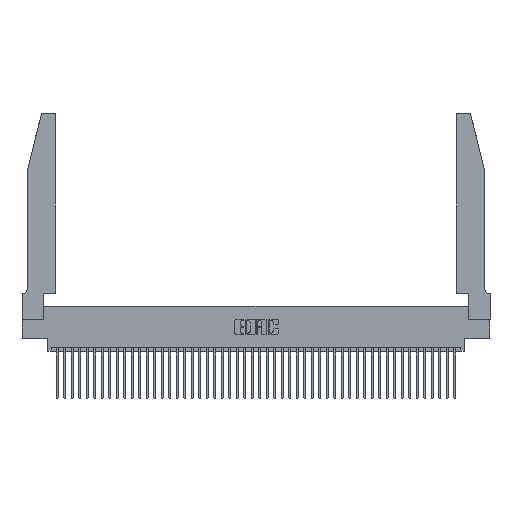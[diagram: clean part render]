
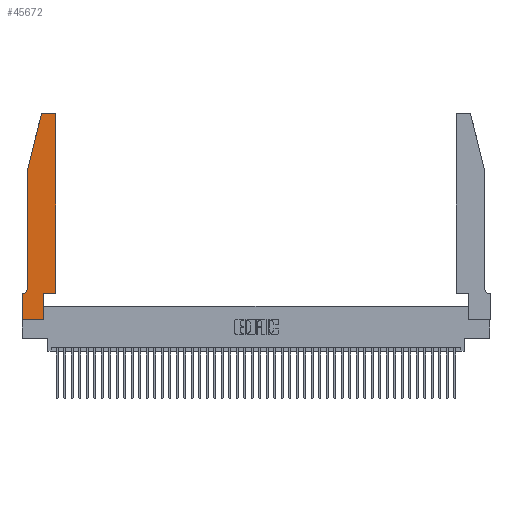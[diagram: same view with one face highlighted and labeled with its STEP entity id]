
A CAD part, top view. The second image highlights one B-rep face of the part: STEP entity #45672.
In plain terms, the highlighted planar face has unit normal (0, 0, 1).
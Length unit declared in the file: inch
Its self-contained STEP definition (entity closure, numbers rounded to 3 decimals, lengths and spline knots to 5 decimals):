
#486 = CARTESIAN_POINT ( 'NONE',  ( 0., 0., 0.37 ) ) ;
#1083 = EDGE_CURVE ( 'NONE', #6959, #23829, #30853, .T. ) ;
#2503 = EDGE_CURVE ( 'NONE', #8473, #39473, #43891, .T. ) ;
#3079 = VECTOR ( 'NONE', #40499, 39.37008 ) ;
#3240 = VECTOR ( 'NONE', #13297, 39.37008 ) ;
#3268 = CARTESIAN_POINT ( 'NONE',  ( 0.2865, 0.35, 0.37 ) ) ;
#3843 = VERTEX_POINT ( 'NONE', #38081 ) ;
#4123 = DIRECTION ( 'NONE',  ( 0., 0., 1. ) ) ;
#4501 = DIRECTION ( 'NONE',  ( 0., 1., 0. ) ) ;
#4898 = DIRECTION ( 'NONE',  ( 0., 0., 1. ) ) ;
#5980 = CIRCLE ( 'NONE', #31203, 0.03 ) ;
#6300 = CARTESIAN_POINT ( 'NONE',  ( 0.4505, 0.35, 0.37 ) ) ;
#6959 = VERTEX_POINT ( 'NONE', #23386 ) ;
#7215 = LINE ( 'NONE', #486, #8301 ) ;
#7235 = ORIENTED_EDGE ( 'NONE', *, *, #12896, .T. ) ;
#7836 = LINE ( 'NONE', #43826, #33857 ) ;
#8301 = VECTOR ( 'NONE', #25407, 39.37008 ) ;
#8470 = VERTEX_POINT ( 'NONE', #41294 ) ;
#8473 = VERTEX_POINT ( 'NONE', #44791 ) ;
#8575 = CIRCLE ( 'NONE', #23532, 0.07 ) ;
#8581 = DIRECTION ( 'NONE',  ( 1., 0., 0. ) ) ;
#10200 = CARTESIAN_POINT ( 'NONE',  ( 0.0055, 0.42, 0.37 ) ) ;
#10315 = CARTESIAN_POINT ( 'NONE',  ( 0.4205, 2.72, 0.37 ) ) ;
#11049 = ORIENTED_EDGE ( 'NONE', *, *, #39092, .T. ) ;
#11539 = CARTESIAN_POINT ( 'NONE',  ( 0.4505, 0.35, 0.37 ) ) ;
#11568 = VERTEX_POINT ( 'NONE', #30779 ) ;
#11853 = EDGE_CURVE ( 'NONE', #8470, #6959, #7215, .T. ) ;
#12227 = ORIENTED_EDGE ( 'NONE', *, *, #2503, .T. ) ;
#12476 = CARTESIAN_POINT ( 'NONE',  ( 0.0755, 2., 0.37 ) ) ;
#12571 = LINE ( 'NONE', #23096, #3079 ) ;
#12896 = EDGE_CURVE ( 'NONE', #3843, #8473, #5980, .T. ) ;
#13297 = DIRECTION ( 'NONE',  ( 0., -1., 0. ) ) ;
#13817 = DIRECTION ( 'NONE',  ( -1., 0., 0. ) ) ;
#13918 = DIRECTION ( 'NONE',  ( 1., 0., 0. ) ) ;
#14577 = VERTEX_POINT ( 'NONE', #24544 ) ;
#15657 = ORIENTED_EDGE ( 'NONE', *, *, #23990, .T. ) ;
#15707 = ORIENTED_EDGE ( 'NONE', *, *, #1083, .T. ) ;
#15874 = ORIENTED_EDGE ( 'NONE', *, *, #19607, .T. ) ;
#16760 = ORIENTED_EDGE ( 'NONE', *, *, #30900, .T. ) ;
#16926 = VERTEX_POINT ( 'NONE', #24470 ) ;
#18142 = VERTEX_POINT ( 'NONE', #6300 ) ;
#19177 = ORIENTED_EDGE ( 'NONE', *, *, #28438, .T. ) ;
#19607 = EDGE_CURVE ( 'NONE', #31777, #8470, #12571, .T. ) ;
#21502 = VECTOR ( 'NONE', #28992, 39.37008 ) ;
#22812 = CIRCLE ( 'NONE', #43787, 0.03 ) ;
#23096 = CARTESIAN_POINT ( 'NONE',  ( 0.0755, 0.35, 0.37 ) ) ;
#23386 = CARTESIAN_POINT ( 'NONE',  ( 0., 0., 0.37 ) ) ;
#23532 = AXIS2_PLACEMENT_3D ( 'NONE', #10200, #34922, #13817 ) ;
#23829 = VERTEX_POINT ( 'NONE', #42460 ) ;
#23990 = EDGE_CURVE ( 'NONE', #18142, #16926, #36699, .T. ) ;
#24232 = LINE ( 'NONE', #43888, #39510 ) ;
#24470 = CARTESIAN_POINT ( 'NONE',  ( 0.4505, 2.72, 0.37 ) ) ;
#24516 = EDGE_CURVE ( 'NONE', #11568, #3843, #26936, .T. ) ;
#24544 = CARTESIAN_POINT ( 'NONE',  ( 0.0755, 0.42, 0.37 ) ) ;
#24729 = ORIENTED_EDGE ( 'NONE', *, *, #42076, .T. ) ;
#25407 = DIRECTION ( 'NONE',  ( 0., -1., 0. ) ) ;
#25462 = CARTESIAN_POINT ( 'NONE',  ( 0.284, 2.72, 0.37 ) ) ;
#26104 = ORIENTED_EDGE ( 'NONE', *, *, #24516, .T. ) ;
#26222 = CARTESIAN_POINT ( 'NONE',  ( 0., 0.35, 0.37 ) ) ;
#26522 = DIRECTION ( 'NONE',  ( 0., 1., 0. ) ) ;
#26936 = LINE ( 'NONE', #42088, #36205 ) ;
#27154 = EDGE_CURVE ( 'NONE', #16926, #11568, #22812, .T. ) ;
#27452 = VECTOR ( 'NONE', #4501, 39.37008 ) ;
#28304 = CARTESIAN_POINT ( 'NONE',  ( 0.0755, 2., 0.37 ) ) ;
#28438 = EDGE_CURVE ( 'NONE', #14577, #31777, #8575, .T. ) ;
#28956 = DIRECTION ( 'NONE',  ( 1., 0., 0. ) ) ;
#28992 = DIRECTION ( 'NONE',  ( 1., 0., 0. ) ) ;
#29713 = DIRECTION ( 'NONE',  ( 1., 0., 0. ) ) ;
#29716 = VERTEX_POINT ( 'NONE', #3268 ) ;
#29879 = ORIENTED_EDGE ( 'NONE', *, *, #11853, .T. ) ;
#30425 = LINE ( 'NONE', #34403, #3240 ) ;
#30736 = AXIS2_PLACEMENT_3D ( 'NONE', #26222, #4898, #29713 ) ;
#30779 = CARTESIAN_POINT ( 'NONE',  ( 0.4205, 2.75, 0.37 ) ) ;
#30853 = LINE ( 'NONE', #42860, #21502 ) ;
#30900 = EDGE_CURVE ( 'NONE', #29716, #18142, #7836, .T. ) ;
#31203 = AXIS2_PLACEMENT_3D ( 'NONE', #25462, #4123, #28956 ) ;
#31777 = VERTEX_POINT ( 'NONE', #44827 ) ;
#33857 = VECTOR ( 'NONE', #8581, 39.37008 ) ;
#34403 = CARTESIAN_POINT ( 'NONE',  ( 0.0755, 2., 0.37 ) ) ;
#34654 = VECTOR ( 'NONE', #44104, 39.37008 ) ;
#34922 = DIRECTION ( 'NONE',  ( 0., 0., -1. ) ) ;
#34933 = ORIENTED_EDGE ( 'NONE', *, *, #27154, .T. ) ;
#35027 = DIRECTION ( 'NONE',  ( 0., 0., 1. ) ) ;
#35277 = DIRECTION ( 'NONE',  ( -1., 0., 0. ) ) ;
#36205 = VECTOR ( 'NONE', #35277, 39.37008 ) ;
#36601 = EDGE_LOOP ( 'NONE', ( #26104, #7235, #12227, #24729, #19177, #15874, #29879, #15707, #11049, #16760, #15657, #34933 ) ) ;
#36699 = LINE ( 'NONE', #11539, #27452 ) ;
#38081 = CARTESIAN_POINT ( 'NONE',  ( 0.284, 2.75, 0.37 ) ) ;
#39092 = EDGE_CURVE ( 'NONE', #23829, #29716, #24232, .T. ) ;
#39473 = VERTEX_POINT ( 'NONE', #28304 ) ;
#39510 = VECTOR ( 'NONE', #26522, 39.37008 ) ;
#40499 = DIRECTION ( 'NONE',  ( -1., 0., 0. ) ) ;
#41294 = CARTESIAN_POINT ( 'NONE',  ( 0., 0.35, 0.37 ) ) ;
#41518 = FACE_OUTER_BOUND ( 'NONE', #36601, .T. ) ;
#42076 = EDGE_CURVE ( 'NONE', #39473, #14577, #30425, .T. ) ;
#42088 = CARTESIAN_POINT ( 'NONE',  ( 0.2605, 2.75, 0.37 ) ) ;
#42460 = CARTESIAN_POINT ( 'NONE',  ( 0.2865, 0., 0.37 ) ) ;
#42860 = CARTESIAN_POINT ( 'NONE',  ( 0., 0., 0.37 ) ) ;
#43571 = PLANE ( 'NONE',  #30736 ) ;
#43787 = AXIS2_PLACEMENT_3D ( 'NONE', #10315, #35027, #13918 ) ;
#43826 = CARTESIAN_POINT ( 'NONE',  ( 0.4505, 0.35, 0.37 ) ) ;
#43888 = CARTESIAN_POINT ( 'NONE',  ( 0.2865, 0.35, 0.37 ) ) ;
#43891 = LINE ( 'NONE', #12476, #34654 ) ;
#44104 = DIRECTION ( 'NONE',  ( -0.239, -0.971, 0. ) ) ;
#44791 = CARTESIAN_POINT ( 'NONE',  ( 0.25487, 2.72718, 0.37 ) ) ;
#44827 = CARTESIAN_POINT ( 'NONE',  ( 0.0055, 0.35, 0.37 ) ) ;
#45672 = ADVANCED_FACE ( 'NONE', ( #41518 ), #43571, .T. ) ;
